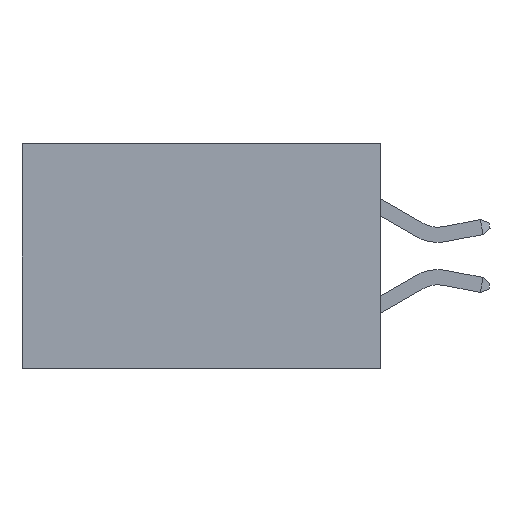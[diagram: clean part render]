
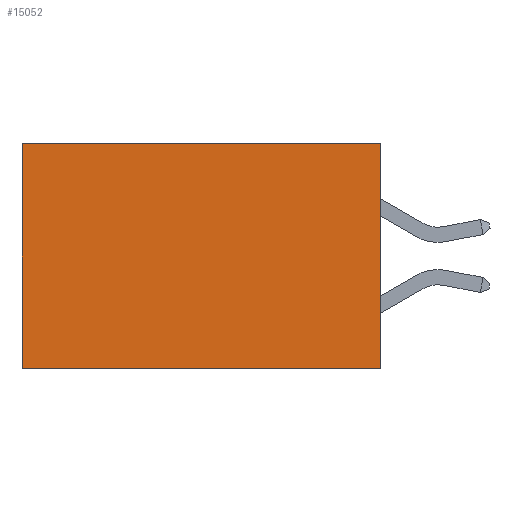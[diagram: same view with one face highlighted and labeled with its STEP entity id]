
A CAD part, left-side view. The second image highlights one B-rep face of the part: STEP entity #15052.
In plain terms, the highlighted planar face has unit normal (-1, 0, 0).
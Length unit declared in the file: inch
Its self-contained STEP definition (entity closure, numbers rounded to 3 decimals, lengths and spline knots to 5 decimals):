
#439 = VERTEX_POINT ( 'NONE', #6284 ) ;
#1068 = CARTESIAN_POINT ( 'NONE',  ( 0.277, 0.59, -0.37 ) ) ;
#1233 = VECTOR ( 'NONE', #5702, 39.37008 ) ;
#1494 = CARTESIAN_POINT ( 'NONE',  ( 0.277, 0., 0. ) ) ;
#2209 = EDGE_CURVE ( 'NONE', #7367, #439, #17114, .T. ) ;
#2420 = DIRECTION ( 'NONE',  ( 0., 1., 0. ) ) ;
#3576 = CARTESIAN_POINT ( 'NONE',  ( 0.277, 0., -0.37 ) ) ;
#4014 = CARTESIAN_POINT ( 'NONE',  ( 0.277, 0.59, -0.37 ) ) ;
#4147 = ORIENTED_EDGE ( 'NONE', *, *, #9087, .T. ) ;
#4849 = DIRECTION ( 'NONE',  ( 1., 0., 0. ) ) ;
#5231 = DIRECTION ( 'NONE',  ( 0., 0., -1. ) ) ;
#5620 = LINE ( 'NONE', #15520, #8915 ) ;
#5638 = LINE ( 'NONE', #4014, #1233 ) ;
#5702 = DIRECTION ( 'NONE',  ( 0., 0., -1. ) ) ;
#6284 = CARTESIAN_POINT ( 'NONE',  ( 0.277, 0.59, 0. ) ) ;
#7367 = VERTEX_POINT ( 'NONE', #1494 ) ;
#7844 = FACE_OUTER_BOUND ( 'NONE', #18290, .T. ) ;
#7870 = EDGE_CURVE ( 'NONE', #11899, #18597, #5620, .T. ) ;
#8345 = CARTESIAN_POINT ( 'NONE',  ( 0.277, 0., 0. ) ) ;
#8915 = VECTOR ( 'NONE', #15252, 39.37008 ) ;
#9087 = EDGE_CURVE ( 'NONE', #439, #18597, #5638, .T. ) ;
#9496 = ORIENTED_EDGE ( 'NONE', *, *, #2209, .T. ) ;
#9573 = EDGE_CURVE ( 'NONE', #7367, #11899, #18787, .T. ) ;
#10431 = VECTOR ( 'NONE', #5231, 39.37008 ) ;
#11322 = CARTESIAN_POINT ( 'NONE',  ( 0.277, 0., -0.37 ) ) ;
#11899 = VERTEX_POINT ( 'NONE', #20262 ) ;
#12760 = ORIENTED_EDGE ( 'NONE', *, *, #7870, .F. ) ;
#14483 = PLANE ( 'NONE',  #16996 ) ;
#14645 = VECTOR ( 'NONE', #2420, 39.37008 ) ;
#15052 = ADVANCED_FACE ( 'NONE', ( #7844 ), #14483, .F. ) ;
#15252 = DIRECTION ( 'NONE',  ( 0., 1., 0. ) ) ;
#15520 = CARTESIAN_POINT ( 'NONE',  ( 0.277, 0., -0.37 ) ) ;
#16079 = DIRECTION ( 'NONE',  ( 0., 0., -1. ) ) ;
#16996 = AXIS2_PLACEMENT_3D ( 'NONE', #11322, #4849, #16079 ) ;
#17114 = LINE ( 'NONE', #8345, #14645 ) ;
#17429 = ORIENTED_EDGE ( 'NONE', *, *, #9573, .F. ) ;
#18290 = EDGE_LOOP ( 'NONE', ( #4147, #12760, #17429, #9496 ) ) ;
#18597 = VERTEX_POINT ( 'NONE', #1068 ) ;
#18787 = LINE ( 'NONE', #3576, #10431 ) ;
#20262 = CARTESIAN_POINT ( 'NONE',  ( 0.277, 0., -0.37 ) ) ;
